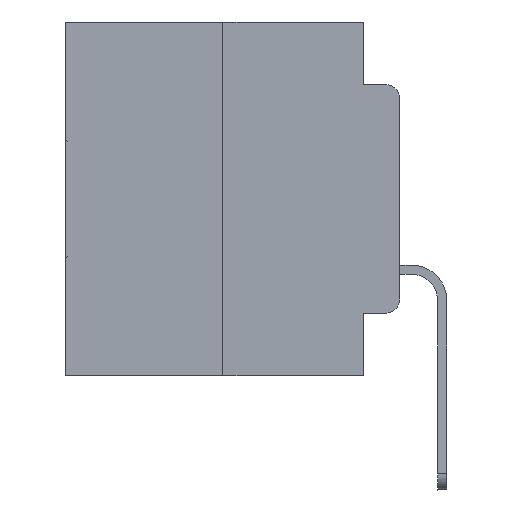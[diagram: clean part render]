
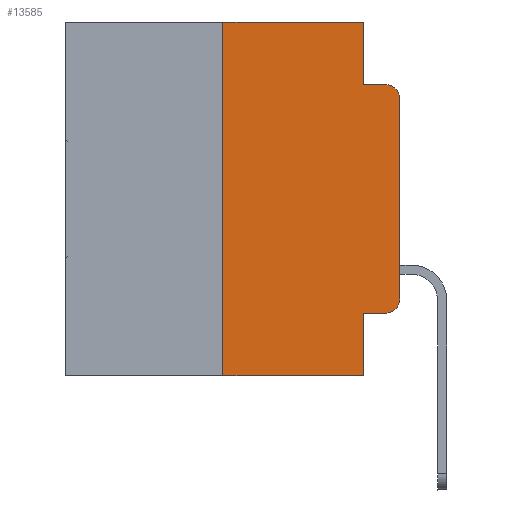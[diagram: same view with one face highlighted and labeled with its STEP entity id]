
A CAD part, left-side view. The second image highlights one B-rep face of the part: STEP entity #13585.
In plain terms, the highlighted planar face has unit normal (-1, 0, 0).
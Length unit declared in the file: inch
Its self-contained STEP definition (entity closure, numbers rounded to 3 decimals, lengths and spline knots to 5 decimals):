
#546 = CARTESIAN_POINT ( 'NONE',  ( 0., 0.051, -0.4115 ) ) ;
#927 = ORIENTED_EDGE ( 'NONE', *, *, #17724, .F. ) ;
#1161 = EDGE_CURVE ( 'NONE', #24794, #25077, #12608, .T. ) ;
#1463 = CARTESIAN_POINT ( 'NONE',  ( 0., 0.25, 0. ) ) ;
#1469 = DIRECTION ( 'NONE',  ( 0., 0., -1. ) ) ;
#1747 = DIRECTION ( 'NONE',  ( 0., -1., 0. ) ) ;
#1812 = ORIENTED_EDGE ( 'NONE', *, *, #20254, .T. ) ;
#2413 = DIRECTION ( 'NONE',  ( 0., 0., -1. ) ) ;
#2855 = ORIENTED_EDGE ( 'NONE', *, *, #19119, .T. ) ;
#3863 = ORIENTED_EDGE ( 'NONE', *, *, #10531, .F. ) ;
#3889 = CARTESIAN_POINT ( 'NONE',  ( 0., 0.051, -0.5 ) ) ;
#3945 = ORIENTED_EDGE ( 'NONE', *, *, #10986, .F. ) ;
#4016 = VERTEX_POINT ( 'NONE', #15729 ) ;
#4066 = LINE ( 'NONE', #1463, #26380 ) ;
#4311 = FACE_OUTER_BOUND ( 'NONE', #16011, .T. ) ;
#4377 = DIRECTION ( 'NONE',  ( 0., -1., 0. ) ) ;
#5344 = DIRECTION ( 'NONE',  ( 0., -1., 0. ) ) ;
#5387 = EDGE_CURVE ( 'NONE', #19698, #23984, #14557, .T. ) ;
#6041 = AXIS2_PLACEMENT_3D ( 'NONE', #8011, #10045, #1469 ) ;
#6308 = VERTEX_POINT ( 'NONE', #13111 ) ;
#7966 = CARTESIAN_POINT ( 'NONE',  ( 0., 0.473, 0. ) ) ;
#8011 = CARTESIAN_POINT ( 'NONE',  ( 0., 0.02, -0.3915 ) ) ;
#9014 = CARTESIAN_POINT ( 'NONE',  ( 0., 0., -0.3915 ) ) ;
#9078 = EDGE_CURVE ( 'NONE', #20036, #28333, #19655, .T. ) ;
#9925 = CARTESIAN_POINT ( 'NONE',  ( 0., 0.051, 0. ) ) ;
#10045 = DIRECTION ( 'NONE',  ( -1., 0., 0. ) ) ;
#10420 = VECTOR ( 'NONE', #16598, 39.37008 ) ;
#10531 = EDGE_CURVE ( 'NONE', #20036, #16992, #27358, .T. ) ;
#10986 = EDGE_CURVE ( 'NONE', #25077, #26520, #18294, .T. ) ;
#11035 = ORIENTED_EDGE ( 'NONE', *, *, #1161, .F. ) ;
#11113 = CARTESIAN_POINT ( 'NONE',  ( 0., 0.473, 0. ) ) ;
#11149 = VECTOR ( 'NONE', #28070, 39.37008 ) ;
#11260 = PLANE ( 'NONE',  #11725 ) ;
#11561 = CIRCLE ( 'NONE', #25304, 0.02 ) ;
#11725 = AXIS2_PLACEMENT_3D ( 'NONE', #11113, #19727, #2413 ) ;
#12608 = LINE ( 'NONE', #7966, #11149 ) ;
#12928 = CARTESIAN_POINT ( 'NONE',  ( 0., 0.051, -0.0885 ) ) ;
#13107 = CARTESIAN_POINT ( 'NONE',  ( 0., 0.051, -0.0885 ) ) ;
#13111 = CARTESIAN_POINT ( 'NONE',  ( 0., 0.02, -0.0885 ) ) ;
#13585 = ADVANCED_FACE ( 'NONE', ( #4311 ), #11260, .F. ) ;
#13663 = CARTESIAN_POINT ( 'NONE',  ( 0., 0.051, 0. ) ) ;
#14557 = LINE ( 'NONE', #18931, #10420 ) ;
#15180 = CARTESIAN_POINT ( 'NONE',  ( 0., 0.25, 0. ) ) ;
#15501 = ORIENTED_EDGE ( 'NONE', *, *, #19444, .T. ) ;
#15539 = CARTESIAN_POINT ( 'NONE',  ( 0., 0.051, 0. ) ) ;
#15729 = CARTESIAN_POINT ( 'NONE',  ( 0., 0.25, -0.5 ) ) ;
#16011 = EDGE_LOOP ( 'NONE', ( #19726, #2855, #25046, #3945, #11035, #927, #1812, #3863, #16967, #15501 ) ) ;
#16103 = VECTOR ( 'NONE', #24548, 39.37008 ) ;
#16598 = DIRECTION ( 'NONE',  ( 0., 0., 1. ) ) ;
#16878 = VECTOR ( 'NONE', #1747, 39.37008 ) ;
#16967 = ORIENTED_EDGE ( 'NONE', *, *, #9078, .T. ) ;
#16992 = VERTEX_POINT ( 'NONE', #3889 ) ;
#17724 = EDGE_CURVE ( 'NONE', #4016, #24794, #4066, .T. ) ;
#17941 = VECTOR ( 'NONE', #25161, 39.37008 ) ;
#18294 = LINE ( 'NONE', #15539, #16103 ) ;
#18736 = CARTESIAN_POINT ( 'NONE',  ( 0., 0.473, -0.5 ) ) ;
#18931 = CARTESIAN_POINT ( 'NONE',  ( 0., 0., 0. ) ) ;
#19119 = EDGE_CURVE ( 'NONE', #23984, #6308, #11561, .T. ) ;
#19444 = EDGE_CURVE ( 'NONE', #28333, #19698, #28356, .T. ) ;
#19655 = LINE ( 'NONE', #21680, #26583 ) ;
#19698 = VERTEX_POINT ( 'NONE', #9014 ) ;
#19726 = ORIENTED_EDGE ( 'NONE', *, *, #5387, .T. ) ;
#19727 = DIRECTION ( 'NONE',  ( 1., 0., 0. ) ) ;
#20036 = VERTEX_POINT ( 'NONE', #546 ) ;
#20254 = EDGE_CURVE ( 'NONE', #4016, #16992, #25275, .T. ) ;
#21680 = CARTESIAN_POINT ( 'NONE',  ( 0., 0.051, -0.4115 ) ) ;
#21707 = DIRECTION ( 'NONE',  ( -1., 0., 0. ) ) ;
#21847 = DIRECTION ( 'NONE',  ( 0., 0., -1. ) ) ;
#22791 = VECTOR ( 'NONE', #5344, 39.37008 ) ;
#23984 = VERTEX_POINT ( 'NONE', #24017 ) ;
#23996 = LINE ( 'NONE', #12928, #16878 ) ;
#24017 = CARTESIAN_POINT ( 'NONE',  ( 0., 0., -0.1085 ) ) ;
#24057 = CARTESIAN_POINT ( 'NONE',  ( 0., 0.02, -0.4115 ) ) ;
#24136 = DIRECTION ( 'NONE',  ( 0., 0., 1. ) ) ;
#24323 = CARTESIAN_POINT ( 'NONE',  ( 0., 0.02, -0.1085 ) ) ;
#24548 = DIRECTION ( 'NONE',  ( 0., 0., -1. ) ) ;
#24794 = VERTEX_POINT ( 'NONE', #15180 ) ;
#25046 = ORIENTED_EDGE ( 'NONE', *, *, #26937, .F. ) ;
#25077 = VERTEX_POINT ( 'NONE', #9925 ) ;
#25161 = DIRECTION ( 'NONE',  ( 0., 0., -1. ) ) ;
#25275 = LINE ( 'NONE', #18736, #22791 ) ;
#25304 = AXIS2_PLACEMENT_3D ( 'NONE', #24323, #21707, #21847 ) ;
#26380 = VECTOR ( 'NONE', #24136, 39.37008 ) ;
#26520 = VERTEX_POINT ( 'NONE', #13107 ) ;
#26583 = VECTOR ( 'NONE', #4377, 39.37008 ) ;
#26937 = EDGE_CURVE ( 'NONE', #26520, #6308, #23996, .T. ) ;
#27358 = LINE ( 'NONE', #13663, #17941 ) ;
#28070 = DIRECTION ( 'NONE',  ( 0., -1., 0. ) ) ;
#28333 = VERTEX_POINT ( 'NONE', #24057 ) ;
#28356 = CIRCLE ( 'NONE', #6041, 0.02 ) ;
